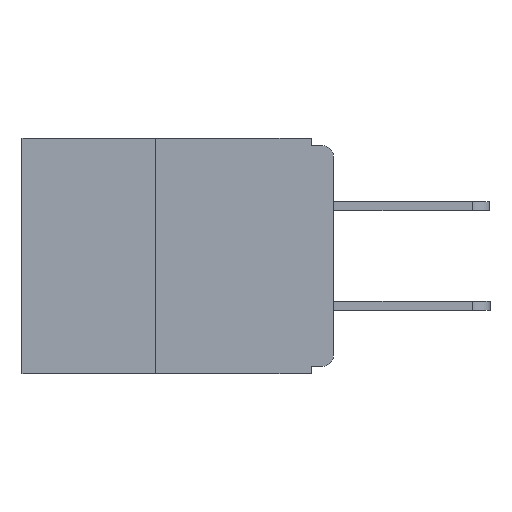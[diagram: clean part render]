
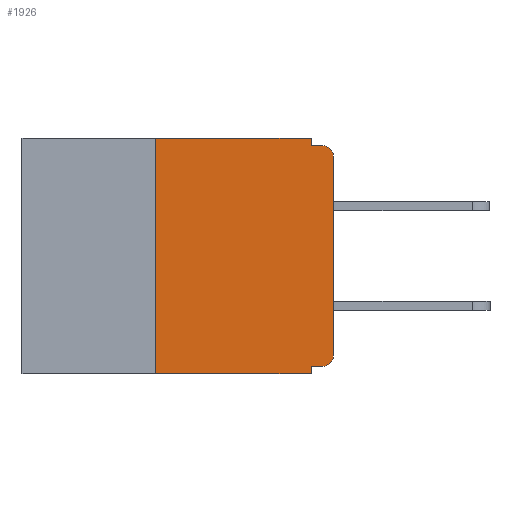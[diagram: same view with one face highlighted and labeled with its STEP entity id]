
A CAD part, left-side view. The second image highlights one B-rep face of the part: STEP entity #1926.
In plain terms, the highlighted planar face has unit normal (-1, 0, 0).
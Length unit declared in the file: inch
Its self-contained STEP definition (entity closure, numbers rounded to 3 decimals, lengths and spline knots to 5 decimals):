
#280 = EDGE_CURVE ( 'NONE', #6059, #7980, #8830, .T. ) ;
#320 = CARTESIAN_POINT ( 'NONE',  ( 0., 0., -0.025 ) ) ;
#401 = VECTOR ( 'NONE', #13790, 39.37008 ) ;
#425 = DIRECTION ( 'NONE',  ( 0., -1., 0. ) ) ;
#606 = CARTESIAN_POINT ( 'NONE',  ( 0., 0.015, -0.01 ) ) ;
#886 = VERTEX_POINT ( 'NONE', #7853 ) ;
#1413 = EDGE_CURVE ( 'NONE', #4787, #14372, #6643, .T. ) ;
#1439 = DIRECTION ( 'NONE',  ( 0., 0., 1. ) ) ;
#1631 = ORIENTED_EDGE ( 'NONE', *, *, #280, .T. ) ;
#1926 = ADVANCED_FACE ( 'NONE', ( #16601 ), #8629, .F. ) ;
#2405 = DIRECTION ( 'NONE',  ( 0., 0., -1. ) ) ;
#2735 = CIRCLE ( 'NONE', #4052, 0.015 ) ;
#3280 = EDGE_CURVE ( 'NONE', #17086, #886, #12437, .T. ) ;
#3355 = AXIS2_PLACEMENT_3D ( 'NONE', #8617, #8557, #2405 ) ;
#3777 = EDGE_CURVE ( 'NONE', #7980, #10891, #7854, .T. ) ;
#3797 = CARTESIAN_POINT ( 'NONE',  ( 0., 0.031, -0.33 ) ) ;
#4052 = AXIS2_PLACEMENT_3D ( 'NONE', #6736, #6719, #6714 ) ;
#4733 = CARTESIAN_POINT ( 'NONE',  ( 0., 0.25, -0.33 ) ) ;
#4787 = VERTEX_POINT ( 'NONE', #13046 ) ;
#4856 = CARTESIAN_POINT ( 'NONE',  ( 0., 0.25, 0. ) ) ;
#5051 = VECTOR ( 'NONE', #6628, 39.37008 ) ;
#5060 = CARTESIAN_POINT ( 'NONE',  ( 0., 0.031, 0. ) ) ;
#5121 = EDGE_CURVE ( 'NONE', #10891, #9981, #2735, .T. ) ;
#5623 = CARTESIAN_POINT ( 'NONE',  ( 0., 0., -0.305 ) ) ;
#5942 = LINE ( 'NONE', #8511, #12438 ) ;
#6059 = VERTEX_POINT ( 'NONE', #11964 ) ;
#6628 = DIRECTION ( 'NONE',  ( 0., 0., -1. ) ) ;
#6643 = LINE ( 'NONE', #4733, #13537 ) ;
#6714 = DIRECTION ( 'NONE',  ( 0., 0., -1. ) ) ;
#6719 = DIRECTION ( 'NONE',  ( -1., 0., 0. ) ) ;
#6736 = CARTESIAN_POINT ( 'NONE',  ( 0., 0.015, -0.025 ) ) ;
#6997 = EDGE_CURVE ( 'NONE', #6059, #15026, #15654, .T. ) ;
#7062 = LINE ( 'NONE', #3797, #17409 ) ;
#7642 = CARTESIAN_POINT ( 'NONE',  ( 0., 0.437, 0. ) ) ;
#7853 = CARTESIAN_POINT ( 'NONE',  ( 0., 0.031, -0.01 ) ) ;
#7854 = LINE ( 'NONE', #14691, #11105 ) ;
#7980 = VERTEX_POINT ( 'NONE', #5623 ) ;
#8021 = ORIENTED_EDGE ( 'NONE', *, *, #6997, .F. ) ;
#8055 = CARTESIAN_POINT ( 'NONE',  ( 0., 0.031, -0.33 ) ) ;
#8244 = CARTESIAN_POINT ( 'NONE',  ( 0., 0., -0.01 ) ) ;
#8373 = VECTOR ( 'NONE', #14128, 39.37008 ) ;
#8511 = CARTESIAN_POINT ( 'NONE',  ( 0., 0.437, -0.33 ) ) ;
#8557 = DIRECTION ( 'NONE',  ( -1., 0., 0. ) ) ;
#8617 = CARTESIAN_POINT ( 'NONE',  ( 0., 0.015, -0.305 ) ) ;
#8629 = PLANE ( 'NONE',  #15572 ) ;
#8830 = CIRCLE ( 'NONE', #3355, 0.015 ) ;
#9317 = ORIENTED_EDGE ( 'NONE', *, *, #15281, .F. ) ;
#9981 = VERTEX_POINT ( 'NONE', #606 ) ;
#10304 = CARTESIAN_POINT ( 'NONE',  ( 0., 0.437, 0. ) ) ;
#10891 = VERTEX_POINT ( 'NONE', #320 ) ;
#10899 = LINE ( 'NONE', #10304, #14121 ) ;
#11105 = VECTOR ( 'NONE', #12155, 39.37008 ) ;
#11221 = LINE ( 'NONE', #8244, #401 ) ;
#11610 = EDGE_CURVE ( 'NONE', #14372, #17086, #10899, .T. ) ;
#11611 = CARTESIAN_POINT ( 'NONE',  ( 0., 0.031, 0. ) ) ;
#11770 = DIRECTION ( 'NONE',  ( 0., 0., -1. ) ) ;
#11825 = ORIENTED_EDGE ( 'NONE', *, *, #3280, .F. ) ;
#11832 = VERTEX_POINT ( 'NONE', #8055 ) ;
#11964 = CARTESIAN_POINT ( 'NONE',  ( 0., 0.015, -0.32 ) ) ;
#12155 = DIRECTION ( 'NONE',  ( 0., 0., 1. ) ) ;
#12437 = LINE ( 'NONE', #11611, #5051 ) ;
#12438 = VECTOR ( 'NONE', #13982, 39.37008 ) ;
#13046 = CARTESIAN_POINT ( 'NONE',  ( 0., 0.25, -0.33 ) ) ;
#13272 = EDGE_LOOP ( 'NONE', ( #14664, #14459, #9317, #11825, #15637, #13577, #16310, #14566, #8021, #1631 ) ) ;
#13537 = VECTOR ( 'NONE', #1439, 39.37008 ) ;
#13546 = DIRECTION ( 'NONE',  ( 0., 0., -1. ) ) ;
#13577 = ORIENTED_EDGE ( 'NONE', *, *, #1413, .F. ) ;
#13790 = DIRECTION ( 'NONE',  ( 0., -1., 0. ) ) ;
#13982 = DIRECTION ( 'NONE',  ( 0., -1., 0. ) ) ;
#14121 = VECTOR ( 'NONE', #425, 39.37008 ) ;
#14128 = DIRECTION ( 'NONE',  ( 0., 1., 0. ) ) ;
#14199 = CARTESIAN_POINT ( 'NONE',  ( 0., 0., -0.32 ) ) ;
#14372 = VERTEX_POINT ( 'NONE', #4856 ) ;
#14459 = ORIENTED_EDGE ( 'NONE', *, *, #5121, .T. ) ;
#14502 = DIRECTION ( 'NONE',  ( 1., 0., 0. ) ) ;
#14566 = ORIENTED_EDGE ( 'NONE', *, *, #16538, .F. ) ;
#14664 = ORIENTED_EDGE ( 'NONE', *, *, #3777, .T. ) ;
#14691 = CARTESIAN_POINT ( 'NONE',  ( 0., 0., 0. ) ) ;
#15026 = VERTEX_POINT ( 'NONE', #15823 ) ;
#15281 = EDGE_CURVE ( 'NONE', #886, #9981, #11221, .T. ) ;
#15572 = AXIS2_PLACEMENT_3D ( 'NONE', #7642, #14502, #11770 ) ;
#15637 = ORIENTED_EDGE ( 'NONE', *, *, #11610, .F. ) ;
#15654 = LINE ( 'NONE', #14199, #8373 ) ;
#15823 = CARTESIAN_POINT ( 'NONE',  ( 0., 0.031, -0.32 ) ) ;
#16310 = ORIENTED_EDGE ( 'NONE', *, *, #17396, .T. ) ;
#16538 = EDGE_CURVE ( 'NONE', #15026, #11832, #7062, .T. ) ;
#16601 = FACE_OUTER_BOUND ( 'NONE', #13272, .T. ) ;
#17086 = VERTEX_POINT ( 'NONE', #5060 ) ;
#17396 = EDGE_CURVE ( 'NONE', #4787, #11832, #5942, .T. ) ;
#17409 = VECTOR ( 'NONE', #13546, 39.37008 ) ;
